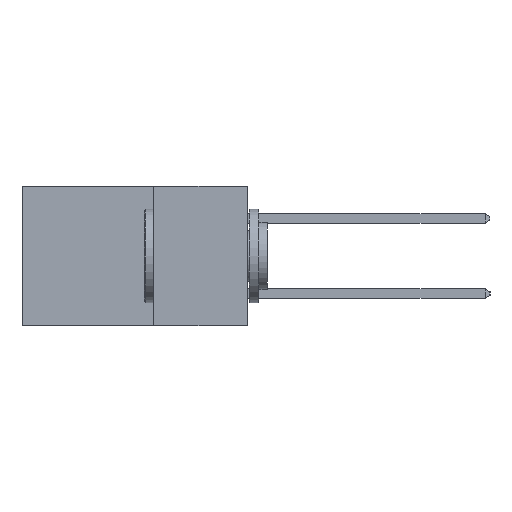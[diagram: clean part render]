
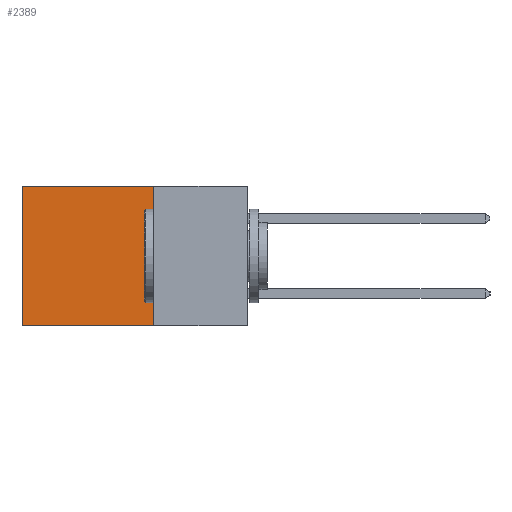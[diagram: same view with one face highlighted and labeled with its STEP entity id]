
A CAD part, left-side view. The second image highlights one B-rep face of the part: STEP entity #2389.
In plain terms, the highlighted planar face has unit normal (-1, 0, 0).
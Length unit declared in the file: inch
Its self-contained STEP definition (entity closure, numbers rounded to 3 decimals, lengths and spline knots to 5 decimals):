
#166 = PLANE ( 'NONE',  #4553 ) ;
#329 = EDGE_LOOP ( 'NONE', ( #4681, #7701, #2511, #4707 ) ) ;
#1714 = CARTESIAN_POINT ( 'NONE',  ( 0.2615, 0.25, -0.37 ) ) ;
#2294 = VECTOR ( 'NONE', #3912, 39.37008 ) ;
#2389 = ADVANCED_FACE ( 'NONE', ( #3254 ), #166, .F. ) ;
#2511 = ORIENTED_EDGE ( 'NONE', *, *, #3625, .F. ) ;
#2609 = CARTESIAN_POINT ( 'NONE',  ( 0.2615, 0.6, -0.37 ) ) ;
#3254 = FACE_OUTER_BOUND ( 'NONE', #329, .T. ) ;
#3598 = DIRECTION ( 'NONE',  ( 0., 0., -1. ) ) ;
#3625 = EDGE_CURVE ( 'NONE', #7414, #7571, #5707, .T. ) ;
#3640 = VERTEX_POINT ( 'NONE', #3823 ) ;
#3823 = CARTESIAN_POINT ( 'NONE',  ( 0.2615, 0.6, 0. ) ) ;
#3912 = DIRECTION ( 'NONE',  ( 0., 0., -1. ) ) ;
#3961 = CARTESIAN_POINT ( 'NONE',  ( 0.2615, 0.25, -0.37 ) ) ;
#4553 = AXIS2_PLACEMENT_3D ( 'NONE', #1714, #12099, #3598 ) ;
#4681 = ORIENTED_EDGE ( 'NONE', *, *, #11213, .T. ) ;
#4707 = ORIENTED_EDGE ( 'NONE', *, *, #11383, .T. ) ;
#4807 = VECTOR ( 'NONE', #12881, 39.37008 ) ;
#5161 = LINE ( 'NONE', #12780, #4807 ) ;
#5707 = LINE ( 'NONE', #3961, #2294 ) ;
#6757 = VECTOR ( 'NONE', #7859, 39.37008 ) ;
#7414 = VERTEX_POINT ( 'NONE', #8956 ) ;
#7571 = VERTEX_POINT ( 'NONE', #11033 ) ;
#7701 = ORIENTED_EDGE ( 'NONE', *, *, #11967, .F. ) ;
#7859 = DIRECTION ( 'NONE',  ( 0., 1., 0. ) ) ;
#8140 = CARTESIAN_POINT ( 'NONE',  ( 0.2615, 0.25, -0.37 ) ) ;
#8956 = CARTESIAN_POINT ( 'NONE',  ( 0.2615, 0.25, 0. ) ) ;
#9713 = LINE ( 'NONE', #8140, #6757 ) ;
#11033 = CARTESIAN_POINT ( 'NONE',  ( 0.2615, 0.25, -0.37 ) ) ;
#11213 = EDGE_CURVE ( 'NONE', #3640, #13547, #5161, .T. ) ;
#11383 = EDGE_CURVE ( 'NONE', #7414, #3640, #11550, .T. ) ;
#11550 = LINE ( 'NONE', #11814, #13715 ) ;
#11796 = DIRECTION ( 'NONE',  ( 0., 1., 0. ) ) ;
#11814 = CARTESIAN_POINT ( 'NONE',  ( 0.2615, 0.25, 0. ) ) ;
#11967 = EDGE_CURVE ( 'NONE', #7571, #13547, #9713, .T. ) ;
#12099 = DIRECTION ( 'NONE',  ( 1., 0., 0. ) ) ;
#12780 = CARTESIAN_POINT ( 'NONE',  ( 0.2615, 0.6, -0.37 ) ) ;
#12881 = DIRECTION ( 'NONE',  ( 0., 0., -1. ) ) ;
#13547 = VERTEX_POINT ( 'NONE', #2609 ) ;
#13715 = VECTOR ( 'NONE', #11796, 39.37008 ) ;
